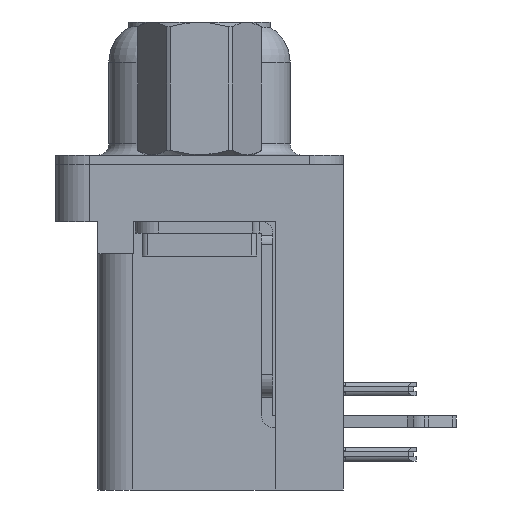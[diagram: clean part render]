
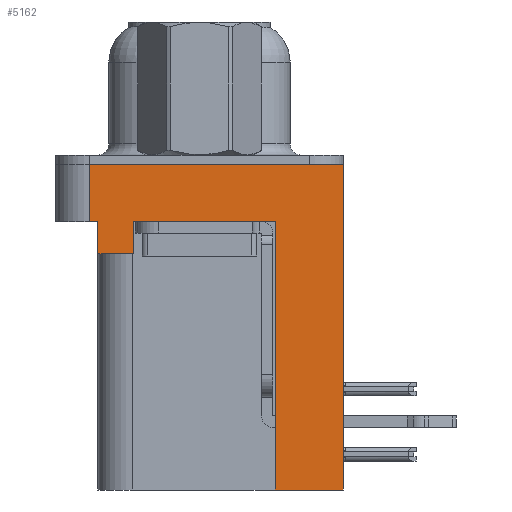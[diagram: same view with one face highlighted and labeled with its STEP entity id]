
A CAD part, left-side view. The second image highlights one B-rep face of the part: STEP entity #5162.
In plain terms, the highlighted planar face has unit normal (-1, 0, 0).
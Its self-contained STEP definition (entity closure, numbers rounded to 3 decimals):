
#650 = DIRECTION ( 'NONE',  ( 0., -1., 0. ) ) ;
#746 = ORIENTED_EDGE ( 'NONE', *, *, #6789, .T. ) ;
#901 = LINE ( 'NONE', #20365, #35002 ) ;
#1191 = EDGE_CURVE ( 'NONE', #23662, #4022, #41459, .T. ) ;
#2048 = CARTESIAN_POINT ( 'NONE',  ( -2.91, -6.275, -2.5 ) ) ;
#2659 = EDGE_CURVE ( 'NONE', #17456, #35983, #6212, .T. ) ;
#4022 = VERTEX_POINT ( 'NONE', #37205 ) ;
#4048 = EDGE_LOOP ( 'NONE', ( #30375, #33789, #39689, #25513, #33561, #5584, #18986, #21623, #24962, #746 ) ) ;
#5006 = FACE_OUTER_BOUND ( 'NONE', #4048, .T. ) ;
#5018 = AXIS2_PLACEMENT_3D ( 'NONE', #2048, #34251, #14337 ) ;
#5162 = ADVANCED_FACE ( 'NONE', ( #5006 ), #17304, .T. ) ;
#5483 = EDGE_CURVE ( 'NONE', #12061, #32437, #25481, .T. ) ;
#5584 = ORIENTED_EDGE ( 'NONE', *, *, #6444, .T. ) ;
#5803 = CARTESIAN_POINT ( 'NONE',  ( -2.91, -6.275, 0. ) ) ;
#6162 = VECTOR ( 'NONE', #10115, 1000. ) ;
#6212 = LINE ( 'NONE', #5803, #26131 ) ;
#6444 = EDGE_CURVE ( 'NONE', #8991, #8994, #28985, .T. ) ;
#6774 = EDGE_CURVE ( 'NONE', #33514, #17456, #15365, .T. ) ;
#6789 = EDGE_CURVE ( 'NONE', #12061, #35983, #18134, .T. ) ;
#8085 = VECTOR ( 'NONE', #16305, 1000. ) ;
#8591 = VECTOR ( 'NONE', #37987, 1000. ) ;
#8991 = VERTEX_POINT ( 'NONE', #39438 ) ;
#8994 = VERTEX_POINT ( 'NONE', #10439 ) ;
#10115 = DIRECTION ( 'NONE',  ( 0., 0., 1. ) ) ;
#10371 = CARTESIAN_POINT ( 'NONE',  ( -2.91, -6.275, -2.5 ) ) ;
#10439 = CARTESIAN_POINT ( 'NONE',  ( -2.91, 2.895, -2.5 ) ) ;
#11722 = CARTESIAN_POINT ( 'NONE',  ( -2.91, -3.295, -14.2 ) ) ;
#12046 = DIRECTION ( 'NONE',  ( 0., 0., 1. ) ) ;
#12061 = VERTEX_POINT ( 'NONE', #27381 ) ;
#12570 = CARTESIAN_POINT ( 'NONE',  ( -2.91, 4.425, -3.9 ) ) ;
#13667 = CARTESIAN_POINT ( 'NONE',  ( -2.91, 4.775, 0. ) ) ;
#14275 = VECTOR ( 'NONE', #12046, 1000. ) ;
#14337 = DIRECTION ( 'NONE',  ( 0., 0., 1. ) ) ;
#15365 = LINE ( 'NONE', #21314, #36404 ) ;
#16305 = DIRECTION ( 'NONE',  ( 0., -1., 0. ) ) ;
#16728 = LINE ( 'NONE', #10371, #8085 ) ;
#16929 = LINE ( 'NONE', #29851, #20032 ) ;
#17224 = EDGE_CURVE ( 'NONE', #8994, #23935, #16929, .T. ) ;
#17304 = PLANE ( 'NONE',  #5018 ) ;
#17456 = VERTEX_POINT ( 'NONE', #13667 ) ;
#17594 = EDGE_CURVE ( 'NONE', #8991, #23662, #18801, .T. ) ;
#18134 = LINE ( 'NONE', #37829, #22228 ) ;
#18732 = DIRECTION ( 'NONE',  ( 0., -1., 0. ) ) ;
#18801 = LINE ( 'NONE', #41016, #41624 ) ;
#18986 = ORIENTED_EDGE ( 'NONE', *, *, #17224, .T. ) ;
#19991 = CARTESIAN_POINT ( 'NONE',  ( -2.91, 4.775, -2.5 ) ) ;
#20032 = VECTOR ( 'NONE', #650, 1000. ) ;
#20365 = CARTESIAN_POINT ( 'NONE',  ( -2.91, -3.295, -14.2 ) ) ;
#21314 = CARTESIAN_POINT ( 'NONE',  ( -2.91, 4.775, -2.5 ) ) ;
#21576 = EDGE_CURVE ( 'NONE', #32437, #23935, #901, .T. ) ;
#21623 = ORIENTED_EDGE ( 'NONE', *, *, #21576, .F. ) ;
#21716 = DIRECTION ( 'NONE',  ( 0., 0., 1. ) ) ;
#22169 = DIRECTION ( 'NONE',  ( 0., 1., 0. ) ) ;
#22228 = VECTOR ( 'NONE', #21716, 1000. ) ;
#23662 = VERTEX_POINT ( 'NONE', #12570 ) ;
#23935 = VERTEX_POINT ( 'NONE', #30763 ) ;
#24962 = ORIENTED_EDGE ( 'NONE', *, *, #5483, .F. ) ;
#25481 = LINE ( 'NONE', #11722, #8591 ) ;
#25513 = ORIENTED_EDGE ( 'NONE', *, *, #1191, .F. ) ;
#26131 = VECTOR ( 'NONE', #18732, 1000. ) ;
#27381 = CARTESIAN_POINT ( 'NONE',  ( -2.91, -6.275, -14.2 ) ) ;
#28041 = EDGE_CURVE ( 'NONE', #33514, #4022, #16728, .T. ) ;
#28985 = LINE ( 'NONE', #29197, #6162 ) ;
#29197 = CARTESIAN_POINT ( 'NONE',  ( -2.91, 2.895, -3.9 ) ) ;
#29851 = CARTESIAN_POINT ( 'NONE',  ( -2.91, -6.275, -2.5 ) ) ;
#30375 = ORIENTED_EDGE ( 'NONE', *, *, #2659, .F. ) ;
#30763 = CARTESIAN_POINT ( 'NONE',  ( -2.91, -3.295, -2.5 ) ) ;
#32437 = VERTEX_POINT ( 'NONE', #33394 ) ;
#33294 = DIRECTION ( 'NONE',  ( 0., 0., 1. ) ) ;
#33394 = CARTESIAN_POINT ( 'NONE',  ( -2.91, -3.295, -14.2 ) ) ;
#33514 = VERTEX_POINT ( 'NONE', #19991 ) ;
#33561 = ORIENTED_EDGE ( 'NONE', *, *, #17594, .F. ) ;
#33789 = ORIENTED_EDGE ( 'NONE', *, *, #6774, .F. ) ;
#34249 = DIRECTION ( 'NONE',  ( 0., 0., 1. ) ) ;
#34251 = DIRECTION ( 'NONE',  ( -1., 0., 0. ) ) ;
#35002 = VECTOR ( 'NONE', #33294, 1000. ) ;
#35983 = VERTEX_POINT ( 'NONE', #36986 ) ;
#36404 = VECTOR ( 'NONE', #34249, 1000. ) ;
#36986 = CARTESIAN_POINT ( 'NONE',  ( -2.91, -6.275, 0. ) ) ;
#37205 = CARTESIAN_POINT ( 'NONE',  ( -2.91, 4.425, -2.5 ) ) ;
#37829 = CARTESIAN_POINT ( 'NONE',  ( -2.91, -6.275, -2.5 ) ) ;
#37987 = DIRECTION ( 'NONE',  ( 0., 1., 0. ) ) ;
#39438 = CARTESIAN_POINT ( 'NONE',  ( -2.91, 2.895, -3.9 ) ) ;
#39689 = ORIENTED_EDGE ( 'NONE', *, *, #28041, .T. ) ;
#41016 = CARTESIAN_POINT ( 'NONE',  ( -2.91, 4.425, -3.9 ) ) ;
#41047 = CARTESIAN_POINT ( 'NONE',  ( -2.91, 4.425, -3.9 ) ) ;
#41459 = LINE ( 'NONE', #41047, #14275 ) ;
#41624 = VECTOR ( 'NONE', #22169, 1000. ) ;
